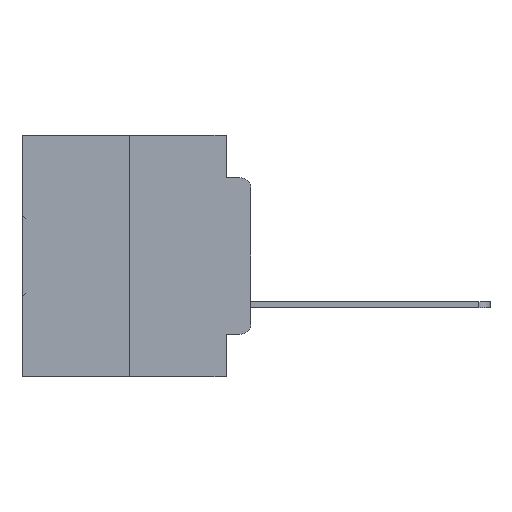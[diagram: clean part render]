
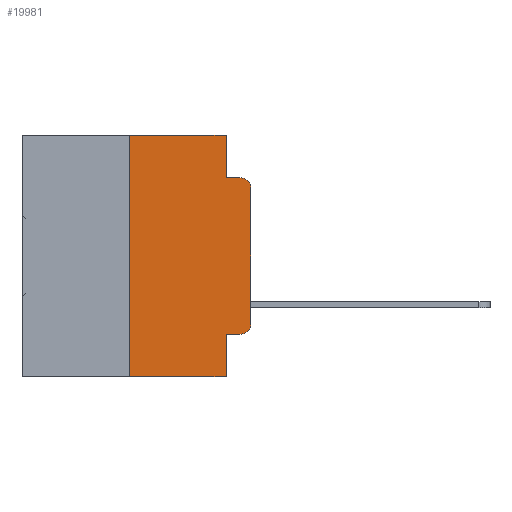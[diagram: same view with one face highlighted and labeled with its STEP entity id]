
A CAD part, left-side view. The second image highlights one B-rep face of the part: STEP entity #19981.
In plain terms, the highlighted planar face has unit normal (-1, 0, 0).
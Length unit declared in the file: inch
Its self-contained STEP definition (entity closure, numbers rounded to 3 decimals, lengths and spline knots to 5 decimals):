
#439 = EDGE_CURVE ( 'NONE', #10845, #2731, #26917, .T. ) ;
#980 = VERTEX_POINT ( 'NONE', #18824 ) ;
#1115 = ORIENTED_EDGE ( 'NONE', *, *, #29613, .T. ) ;
#1784 = CIRCLE ( 'NONE', #12355, 0.02 ) ;
#1980 = ORIENTED_EDGE ( 'NONE', *, *, #5473, .T. ) ;
#2119 = ORIENTED_EDGE ( 'NONE', *, *, #28015, .F. ) ;
#2214 = VECTOR ( 'NONE', #17440, 39.37008 ) ;
#2731 = VERTEX_POINT ( 'NONE', #23924 ) ;
#2771 = DIRECTION ( 'NONE',  ( 0., -1., 0. ) ) ;
#3335 = ORIENTED_EDGE ( 'NONE', *, *, #31221, .T. ) ;
#3672 = DIRECTION ( 'NONE',  ( -1., 0., 0. ) ) ;
#3716 = VERTEX_POINT ( 'NONE', #14549 ) ;
#4174 = CARTESIAN_POINT ( 'NONE',  ( 0., 0.25, 0. ) ) ;
#4457 = CARTESIAN_POINT ( 'NONE',  ( 0., 0.02, -0.0885 ) ) ;
#4676 = VERTEX_POINT ( 'NONE', #12238 ) ;
#4685 = ORIENTED_EDGE ( 'NONE', *, *, #26406, .F. ) ;
#5350 = DIRECTION ( 'NONE',  ( 0., -1., 0. ) ) ;
#5473 = EDGE_CURVE ( 'NONE', #4676, #5561, #19189, .T. ) ;
#5561 = VERTEX_POINT ( 'NONE', #8322 ) ;
#5781 = VECTOR ( 'NONE', #5350, 39.37008 ) ;
#6154 = VECTOR ( 'NONE', #7043, 39.37008 ) ;
#7043 = DIRECTION ( 'NONE',  ( 0., 0., 1. ) ) ;
#7999 = LINE ( 'NONE', #4174, #6154 ) ;
#8256 = ORIENTED_EDGE ( 'NONE', *, *, #24767, .F. ) ;
#8322 = CARTESIAN_POINT ( 'NONE',  ( 0., 0.051, -0.5 ) ) ;
#8346 = CARTESIAN_POINT ( 'NONE',  ( 0., 0.25, 0. ) ) ;
#9049 = LINE ( 'NONE', #32923, #23260 ) ;
#9536 = DIRECTION ( 'NONE',  ( 0., 0., -1. ) ) ;
#9887 = AXIS2_PLACEMENT_3D ( 'NONE', #31658, #34045, #19440 ) ;
#10845 = VERTEX_POINT ( 'NONE', #8346 ) ;
#10971 = VECTOR ( 'NONE', #9536, 39.37008 ) ;
#12238 = CARTESIAN_POINT ( 'NONE',  ( 0., 0.25, -0.5 ) ) ;
#12355 = AXIS2_PLACEMENT_3D ( 'NONE', #31560, #16678, #33930 ) ;
#13795 = CARTESIAN_POINT ( 'NONE',  ( 0., 0.473, 0. ) ) ;
#14072 = ORIENTED_EDGE ( 'NONE', *, *, #19685, .T. ) ;
#14272 = VERTEX_POINT ( 'NONE', #25631 ) ;
#14549 = CARTESIAN_POINT ( 'NONE',  ( 0., 0.051, -0.0885 ) ) ;
#15261 = EDGE_LOOP ( 'NONE', ( #3335, #1115, #2119, #4685, #18557, #8256, #1980, #18636, #14072, #16634 ) ) ;
#16122 = CARTESIAN_POINT ( 'NONE',  ( 0., 0.473, -0.5 ) ) ;
#16157 = EDGE_CURVE ( 'NONE', #29590, #30346, #23706, .T. ) ;
#16259 = DIRECTION ( 'NONE',  ( 0., 0., 1. ) ) ;
#16634 = ORIENTED_EDGE ( 'NONE', *, *, #16157, .T. ) ;
#16678 = DIRECTION ( 'NONE',  ( -1., 0., 0. ) ) ;
#17440 = DIRECTION ( 'NONE',  ( 0., 0., -1. ) ) ;
#17598 = VECTOR ( 'NONE', #2771, 39.37008 ) ;
#18269 = DIRECTION ( 'NONE',  ( 0., -1., 0. ) ) ;
#18557 = ORIENTED_EDGE ( 'NONE', *, *, #439, .F. ) ;
#18636 = ORIENTED_EDGE ( 'NONE', *, *, #21483, .F. ) ;
#18824 = CARTESIAN_POINT ( 'NONE',  ( 0., 0.051, -0.4115 ) ) ;
#18827 = DIRECTION ( 'NONE',  ( 0., -1., 0. ) ) ;
#19189 = LINE ( 'NONE', #16122, #31468 ) ;
#19440 = DIRECTION ( 'NONE',  ( 0., 0., -1. ) ) ;
#19685 = EDGE_CURVE ( 'NONE', #980, #29590, #9049, .T. ) ;
#19981 = ADVANCED_FACE ( 'NONE', ( #27008 ), #29291, .F. ) ;
#20127 = CARTESIAN_POINT ( 'NONE',  ( 0., 0.02, -0.3915 ) ) ;
#21483 = EDGE_CURVE ( 'NONE', #980, #5561, #23943, .T. ) ;
#21870 = CARTESIAN_POINT ( 'NONE',  ( 0., 0.02, -0.4115 ) ) ;
#22343 = AXIS2_PLACEMENT_3D ( 'NONE', #20127, #3672, #22693 ) ;
#22693 = DIRECTION ( 'NONE',  ( 0., 0., -1. ) ) ;
#23260 = VECTOR ( 'NONE', #18269, 39.37008 ) ;
#23706 = CIRCLE ( 'NONE', #22343, 0.02 ) ;
#23924 = CARTESIAN_POINT ( 'NONE',  ( 0., 0.051, 0. ) ) ;
#23943 = LINE ( 'NONE', #29724, #2214 ) ;
#24387 = LINE ( 'NONE', #31626, #17598 ) ;
#24767 = EDGE_CURVE ( 'NONE', #4676, #10845, #7999, .T. ) ;
#25631 = CARTESIAN_POINT ( 'NONE',  ( 0., 0., -0.1085 ) ) ;
#26151 = VECTOR ( 'NONE', #16259, 39.37008 ) ;
#26406 = EDGE_CURVE ( 'NONE', #2731, #3716, #30539, .T. ) ;
#26917 = LINE ( 'NONE', #13795, #5781 ) ;
#27008 = FACE_OUTER_BOUND ( 'NONE', #15261, .T. ) ;
#27734 = CARTESIAN_POINT ( 'NONE',  ( 0., 0.051, 0. ) ) ;
#28015 = EDGE_CURVE ( 'NONE', #3716, #29221, #24387, .T. ) ;
#28835 = CARTESIAN_POINT ( 'NONE',  ( 0., 0., 0. ) ) ;
#29221 = VERTEX_POINT ( 'NONE', #4457 ) ;
#29291 = PLANE ( 'NONE',  #9887 ) ;
#29590 = VERTEX_POINT ( 'NONE', #21870 ) ;
#29613 = EDGE_CURVE ( 'NONE', #14272, #29221, #1784, .T. ) ;
#29724 = CARTESIAN_POINT ( 'NONE',  ( 0., 0.051, 0. ) ) ;
#30346 = VERTEX_POINT ( 'NONE', #33599 ) ;
#30539 = LINE ( 'NONE', #27734, #10971 ) ;
#31221 = EDGE_CURVE ( 'NONE', #30346, #14272, #32462, .T. ) ;
#31468 = VECTOR ( 'NONE', #18827, 39.37008 ) ;
#31560 = CARTESIAN_POINT ( 'NONE',  ( 0., 0.02, -0.1085 ) ) ;
#31626 = CARTESIAN_POINT ( 'NONE',  ( 0., 0.051, -0.0885 ) ) ;
#31658 = CARTESIAN_POINT ( 'NONE',  ( 0., 0.473, 0. ) ) ;
#32462 = LINE ( 'NONE', #28835, #26151 ) ;
#32923 = CARTESIAN_POINT ( 'NONE',  ( 0., 0.051, -0.4115 ) ) ;
#33599 = CARTESIAN_POINT ( 'NONE',  ( 0., 0., -0.3915 ) ) ;
#33930 = DIRECTION ( 'NONE',  ( 0., 0., -1. ) ) ;
#34045 = DIRECTION ( 'NONE',  ( 1., 0., 0. ) ) ;
